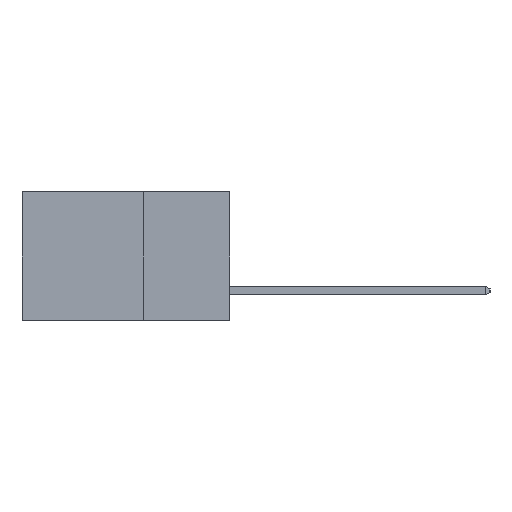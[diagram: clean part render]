
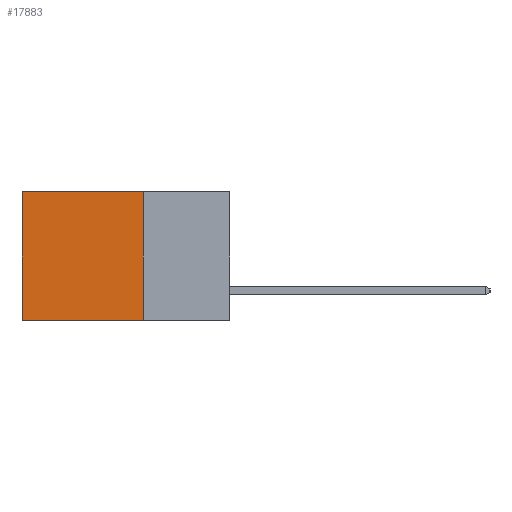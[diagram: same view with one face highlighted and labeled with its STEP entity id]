
A CAD part, left-side view. The second image highlights one B-rep face of the part: STEP entity #17883.
In plain terms, the highlighted planar face has unit normal (-1, 0, 0).
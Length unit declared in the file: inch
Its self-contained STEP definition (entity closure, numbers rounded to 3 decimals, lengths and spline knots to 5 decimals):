
#274 = AXIS2_PLACEMENT_3D ( 'NONE', #18139, #8896, #19607 ) ;
#599 = DIRECTION ( 'NONE',  ( 0., 0., -1. ) ) ;
#695 = EDGE_LOOP ( 'NONE', ( #16889, #17141, #16697, #6698 ) ) ;
#799 = EDGE_CURVE ( 'NONE', #7850, #9000, #6361, .T. ) ;
#1312 = EDGE_CURVE ( 'NONE', #7850, #9199, #14073, .T. ) ;
#1753 = LINE ( 'NONE', #2325, #9346 ) ;
#2325 = CARTESIAN_POINT ( 'NONE',  ( 0.2615, 0.6, -0.37 ) ) ;
#3112 = CARTESIAN_POINT ( 'NONE',  ( 0.2615, 0.6, 0. ) ) ;
#4679 = CARTESIAN_POINT ( 'NONE',  ( 0.2615, 0.25, -0.37 ) ) ;
#5874 = PLANE ( 'NONE',  #274 ) ;
#5906 = VERTEX_POINT ( 'NONE', #6368 ) ;
#6361 = LINE ( 'NONE', #18668, #14107 ) ;
#6368 = CARTESIAN_POINT ( 'NONE',  ( 0.2615, 0.6, -0.37 ) ) ;
#6698 = ORIENTED_EDGE ( 'NONE', *, *, #1312, .T. ) ;
#7276 = FACE_OUTER_BOUND ( 'NONE', #695, .T. ) ;
#7850 = VERTEX_POINT ( 'NONE', #18160 ) ;
#8274 = CARTESIAN_POINT ( 'NONE',  ( 0.2615, 0.25, 0. ) ) ;
#8548 = EDGE_CURVE ( 'NONE', #9000, #5906, #18817, .T. ) ;
#8896 = DIRECTION ( 'NONE',  ( 1., 0., 0. ) ) ;
#9000 = VERTEX_POINT ( 'NONE', #13364 ) ;
#9199 = VERTEX_POINT ( 'NONE', #3112 ) ;
#9346 = VECTOR ( 'NONE', #14531, 39.37008 ) ;
#11869 = DIRECTION ( 'NONE',  ( 0., 1., 0. ) ) ;
#13364 = CARTESIAN_POINT ( 'NONE',  ( 0.2615, 0.25, -0.37 ) ) ;
#13603 = VECTOR ( 'NONE', #11869, 39.37008 ) ;
#13847 = DIRECTION ( 'NONE',  ( 0., 1., 0. ) ) ;
#14073 = LINE ( 'NONE', #8274, #13603 ) ;
#14107 = VECTOR ( 'NONE', #599, 39.37008 ) ;
#14531 = DIRECTION ( 'NONE',  ( 0., 0., -1. ) ) ;
#16697 = ORIENTED_EDGE ( 'NONE', *, *, #799, .F. ) ;
#16889 = ORIENTED_EDGE ( 'NONE', *, *, #19544, .T. ) ;
#17141 = ORIENTED_EDGE ( 'NONE', *, *, #8548, .F. ) ;
#17883 = ADVANCED_FACE ( 'NONE', ( #7276 ), #5874, .F. ) ;
#18139 = CARTESIAN_POINT ( 'NONE',  ( 0.2615, 0.25, -0.37 ) ) ;
#18160 = CARTESIAN_POINT ( 'NONE',  ( 0.2615, 0.25, 0. ) ) ;
#18359 = VECTOR ( 'NONE', #13847, 39.37008 ) ;
#18668 = CARTESIAN_POINT ( 'NONE',  ( 0.2615, 0.25, -0.37 ) ) ;
#18817 = LINE ( 'NONE', #4679, #18359 ) ;
#19544 = EDGE_CURVE ( 'NONE', #9199, #5906, #1753, .T. ) ;
#19607 = DIRECTION ( 'NONE',  ( 0., 0., -1. ) ) ;
